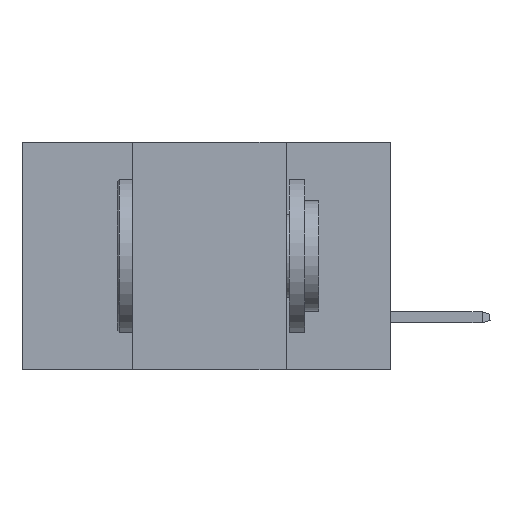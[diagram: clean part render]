
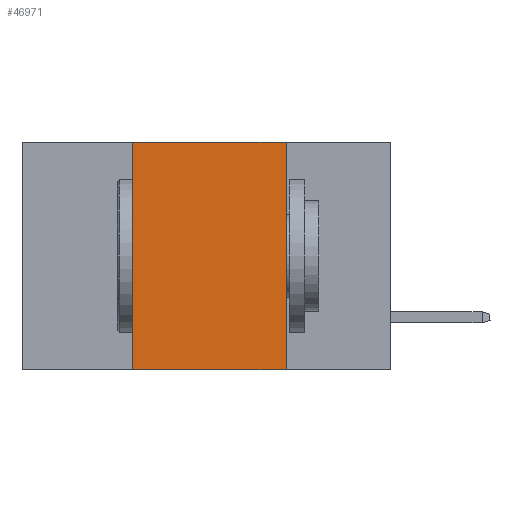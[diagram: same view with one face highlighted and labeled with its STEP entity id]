
A CAD part, left-side view. The second image highlights one B-rep face of the part: STEP entity #46971.
In plain terms, the highlighted planar face has unit normal (-1, 0, 0).
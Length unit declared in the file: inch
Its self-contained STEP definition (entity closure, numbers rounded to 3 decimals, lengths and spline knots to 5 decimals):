
#748 = EDGE_LOOP ( 'NONE', ( #43476, #26241, #30701, #3163 ) ) ;
#777 = CARTESIAN_POINT ( 'NONE',  ( 0., 0.6, -0.37 ) ) ;
#2097 = DIRECTION ( 'NONE',  ( 1., 0., 0. ) ) ;
#2322 = CARTESIAN_POINT ( 'NONE',  ( 0., 0.6, 0. ) ) ;
#2745 = VECTOR ( 'NONE', #21874, 39.37008 ) ;
#2914 = VECTOR ( 'NONE', #3844, 39.37008 ) ;
#3163 = ORIENTED_EDGE ( 'NONE', *, *, #20189, .T. ) ;
#3540 = CARTESIAN_POINT ( 'NONE',  ( 0., 0.17, 0. ) ) ;
#3844 = DIRECTION ( 'NONE',  ( 0., -1., 0. ) ) ;
#5272 = VERTEX_POINT ( 'NONE', #22663 ) ;
#7601 = VECTOR ( 'NONE', #39623, 39.37008 ) ;
#9757 = EDGE_CURVE ( 'NONE', #47224, #5272, #10350, .T. ) ;
#9796 = PLANE ( 'NONE',  #37314 ) ;
#10121 = CARTESIAN_POINT ( 'NONE',  ( 0., 0.6, 0. ) ) ;
#10350 = LINE ( 'NONE', #26383, #43826 ) ;
#18149 = LINE ( 'NONE', #777, #2914 ) ;
#19724 = LINE ( 'NONE', #20227, #7601 ) ;
#19857 = VERTEX_POINT ( 'NONE', #37175 ) ;
#20189 = EDGE_CURVE ( 'NONE', #47224, #19857, #18149, .T. ) ;
#20227 = CARTESIAN_POINT ( 'NONE',  ( 0., 0.17, 0. ) ) ;
#21874 = DIRECTION ( 'NONE',  ( 0., -1., 0. ) ) ;
#22455 = EDGE_CURVE ( 'NONE', #35483, #19857, #19724, .T. ) ;
#22663 = CARTESIAN_POINT ( 'NONE',  ( 0., 0.42, 0. ) ) ;
#26241 = ORIENTED_EDGE ( 'NONE', *, *, #48693, .F. ) ;
#26383 = CARTESIAN_POINT ( 'NONE',  ( 0., 0.42, 0. ) ) ;
#29735 = FACE_OUTER_BOUND ( 'NONE', #748, .T. ) ;
#30701 = ORIENTED_EDGE ( 'NONE', *, *, #9757, .F. ) ;
#35483 = VERTEX_POINT ( 'NONE', #3540 ) ;
#36852 = LINE ( 'NONE', #2322, #2745 ) ;
#37175 = CARTESIAN_POINT ( 'NONE',  ( 0., 0.17, -0.37 ) ) ;
#37303 = DIRECTION ( 'NONE',  ( 0., 0., -1. ) ) ;
#37314 = AXIS2_PLACEMENT_3D ( 'NONE', #10121, #2097, #37303 ) ;
#38638 = CARTESIAN_POINT ( 'NONE',  ( 0., 0.42, -0.37 ) ) ;
#39623 = DIRECTION ( 'NONE',  ( 0., 0., -1. ) ) ;
#43476 = ORIENTED_EDGE ( 'NONE', *, *, #22455, .F. ) ;
#43826 = VECTOR ( 'NONE', #49694, 39.37008 ) ;
#46971 = ADVANCED_FACE ( 'NONE', ( #29735 ), #9796, .F. ) ;
#47224 = VERTEX_POINT ( 'NONE', #38638 ) ;
#48693 = EDGE_CURVE ( 'NONE', #5272, #35483, #36852, .T. ) ;
#49694 = DIRECTION ( 'NONE',  ( 0., 0., 1. ) ) ;
